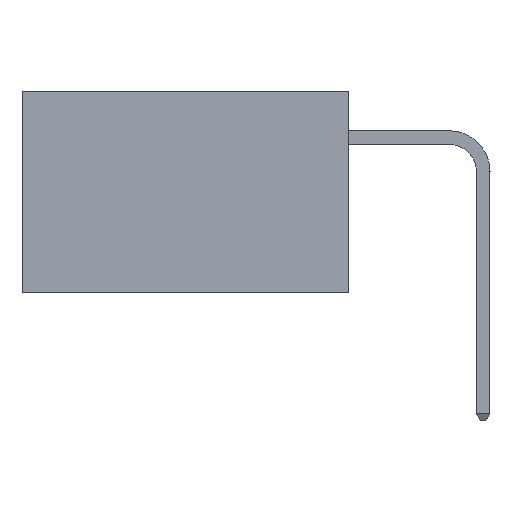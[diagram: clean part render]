
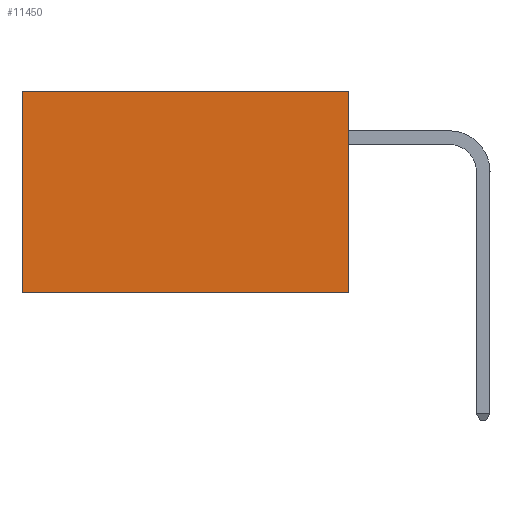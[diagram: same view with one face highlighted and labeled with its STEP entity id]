
A CAD part, left-side view. The second image highlights one B-rep face of the part: STEP entity #11450.
In plain terms, the highlighted planar face has unit normal (-1, 0, 0).
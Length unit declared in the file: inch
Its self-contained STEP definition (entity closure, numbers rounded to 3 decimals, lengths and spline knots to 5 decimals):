
#468 = LINE ( 'NONE', #12249, #16365 ) ;
#902 = DIRECTION ( 'NONE',  ( 0., 0., -1. ) ) ;
#1352 = DIRECTION ( 'NONE',  ( 0., 1., 0. ) ) ;
#2474 = DIRECTION ( 'NONE',  ( 0., 0., -1. ) ) ;
#3856 = CARTESIAN_POINT ( 'NONE',  ( 0.2875, 0.6, 0. ) ) ;
#5035 = PLANE ( 'NONE',  #7120 ) ;
#5339 = CARTESIAN_POINT ( 'NONE',  ( 0.2875, 0., -0.37 ) ) ;
#5551 = VERTEX_POINT ( 'NONE', #18280 ) ;
#5992 = DIRECTION ( 'NONE',  ( 0., 0., -1. ) ) ;
#6204 = EDGE_LOOP ( 'NONE', ( #11144, #16509, #17993, #25640 ) ) ;
#7120 = AXIS2_PLACEMENT_3D ( 'NONE', #7142, #13341, #902 ) ;
#7142 = CARTESIAN_POINT ( 'NONE',  ( 0.2875, 0., 0. ) ) ;
#7904 = VECTOR ( 'NONE', #2474, 39.37008 ) ;
#9521 = EDGE_CURVE ( 'NONE', #14486, #16671, #13378, .T. ) ;
#9765 = FACE_OUTER_BOUND ( 'NONE', #6204, .T. ) ;
#10549 = VECTOR ( 'NONE', #5992, 39.37008 ) ;
#10595 = LINE ( 'NONE', #11745, #20153 ) ;
#11144 = ORIENTED_EDGE ( 'NONE', *, *, #18645, .T. ) ;
#11450 = ADVANCED_FACE ( 'NONE', ( #9765 ), #5035, .F. ) ;
#11745 = CARTESIAN_POINT ( 'NONE',  ( 0.2875, 0., 0. ) ) ;
#12249 = CARTESIAN_POINT ( 'NONE',  ( 0.2875, 0., -0.37 ) ) ;
#13341 = DIRECTION ( 'NONE',  ( 1., 0., 0. ) ) ;
#13378 = LINE ( 'NONE', #22916, #7904 ) ;
#14269 = DIRECTION ( 'NONE',  ( 0., 1., 0. ) ) ;
#14486 = VERTEX_POINT ( 'NONE', #24439 ) ;
#16365 = VECTOR ( 'NONE', #14269, 39.37008 ) ;
#16509 = ORIENTED_EDGE ( 'NONE', *, *, #18020, .F. ) ;
#16671 = VERTEX_POINT ( 'NONE', #5339 ) ;
#17222 = EDGE_CURVE ( 'NONE', #14486, #21969, #10595, .T. ) ;
#17993 = ORIENTED_EDGE ( 'NONE', *, *, #9521, .F. ) ;
#18020 = EDGE_CURVE ( 'NONE', #16671, #5551, #468, .T. ) ;
#18280 = CARTESIAN_POINT ( 'NONE',  ( 0.2875, 0.6, -0.37 ) ) ;
#18645 = EDGE_CURVE ( 'NONE', #21969, #5551, #23228, .T. ) ;
#19991 = CARTESIAN_POINT ( 'NONE',  ( 0.2875, 0.6, 0. ) ) ;
#20153 = VECTOR ( 'NONE', #1352, 39.37008 ) ;
#21969 = VERTEX_POINT ( 'NONE', #19991 ) ;
#22916 = CARTESIAN_POINT ( 'NONE',  ( 0.2875, 0., 0. ) ) ;
#23228 = LINE ( 'NONE', #3856, #10549 ) ;
#24439 = CARTESIAN_POINT ( 'NONE',  ( 0.2875, 0., 0. ) ) ;
#25640 = ORIENTED_EDGE ( 'NONE', *, *, #17222, .T. ) ;
